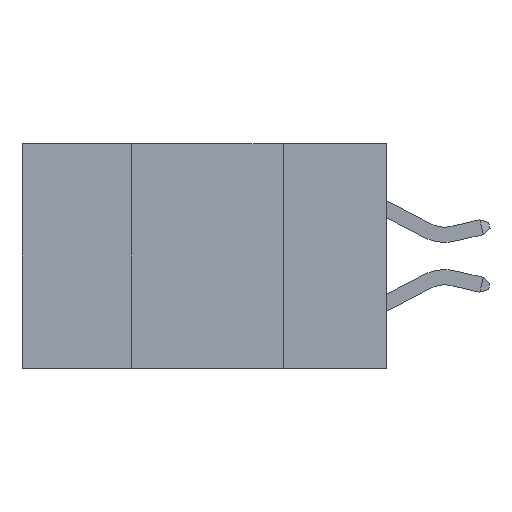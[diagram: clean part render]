
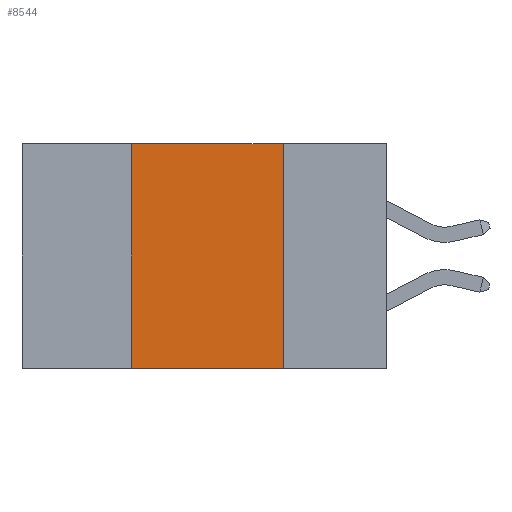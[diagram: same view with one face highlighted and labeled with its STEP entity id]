
A CAD part, left-side view. The second image highlights one B-rep face of the part: STEP entity #8544.
In plain terms, the highlighted planar face has unit normal (-1, 0, 0).
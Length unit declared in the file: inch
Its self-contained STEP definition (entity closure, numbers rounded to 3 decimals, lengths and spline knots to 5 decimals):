
#310 = CARTESIAN_POINT ( 'NONE',  ( 0., 0.17, -0.37 ) ) ;
#622 = DIRECTION ( 'NONE',  ( 0., -1., 0. ) ) ;
#941 = DIRECTION ( 'NONE',  ( 0., -1., 0. ) ) ;
#1132 = LINE ( 'NONE', #11009, #13614 ) ;
#1211 = EDGE_CURVE ( 'NONE', #13807, #11804, #8291, .T. ) ;
#2647 = CARTESIAN_POINT ( 'NONE',  ( 0., 0.42, 0. ) ) ;
#2717 = DIRECTION ( 'NONE',  ( 0., 0., -1. ) ) ;
#3360 = CARTESIAN_POINT ( 'NONE',  ( 0., 0.17, 0. ) ) ;
#3822 = CARTESIAN_POINT ( 'NONE',  ( 0., 0.42, -0.37 ) ) ;
#3830 = ORIENTED_EDGE ( 'NONE', *, *, #1211, .T. ) ;
#4068 = PLANE ( 'NONE',  #12578 ) ;
#4721 = ORIENTED_EDGE ( 'NONE', *, *, #5533, .F. ) ;
#4984 = VECTOR ( 'NONE', #8872, 39.37008 ) ;
#5191 = DIRECTION ( 'NONE',  ( 1., 0., 0. ) ) ;
#5192 = VECTOR ( 'NONE', #941, 39.37008 ) ;
#5195 = VECTOR ( 'NONE', #2717, 39.37008 ) ;
#5358 = CARTESIAN_POINT ( 'NONE',  ( 0., 0.42, 0. ) ) ;
#5402 = ORIENTED_EDGE ( 'NONE', *, *, #12005, .F. ) ;
#5533 = EDGE_CURVE ( 'NONE', #8798, #11804, #7915, .T. ) ;
#7384 = EDGE_CURVE ( 'NONE', #13807, #9056, #8074, .T. ) ;
#7778 = EDGE_LOOP ( 'NONE', ( #4721, #5402, #8867, #3830 ) ) ;
#7915 = LINE ( 'NONE', #9540, #5195 ) ;
#8074 = LINE ( 'NONE', #5358, #4984 ) ;
#8291 = LINE ( 'NONE', #11843, #5192 ) ;
#8544 = ADVANCED_FACE ( 'NONE', ( #10197 ), #4068, .F. ) ;
#8798 = VERTEX_POINT ( 'NONE', #3360 ) ;
#8867 = ORIENTED_EDGE ( 'NONE', *, *, #7384, .F. ) ;
#8872 = DIRECTION ( 'NONE',  ( 0., 0., 1. ) ) ;
#9056 = VERTEX_POINT ( 'NONE', #2647 ) ;
#9540 = CARTESIAN_POINT ( 'NONE',  ( 0., 0.17, 0. ) ) ;
#9800 = CARTESIAN_POINT ( 'NONE',  ( 0., 0.6, 0. ) ) ;
#10197 = FACE_OUTER_BOUND ( 'NONE', #7778, .T. ) ;
#11009 = CARTESIAN_POINT ( 'NONE',  ( 0., 0.6, 0. ) ) ;
#11804 = VERTEX_POINT ( 'NONE', #310 ) ;
#11843 = CARTESIAN_POINT ( 'NONE',  ( 0., 0.6, -0.37 ) ) ;
#12005 = EDGE_CURVE ( 'NONE', #9056, #8798, #1132, .T. ) ;
#12578 = AXIS2_PLACEMENT_3D ( 'NONE', #9800, #5191, #13139 ) ;
#13139 = DIRECTION ( 'NONE',  ( 0., 0., -1. ) ) ;
#13614 = VECTOR ( 'NONE', #622, 39.37008 ) ;
#13807 = VERTEX_POINT ( 'NONE', #3822 ) ;
